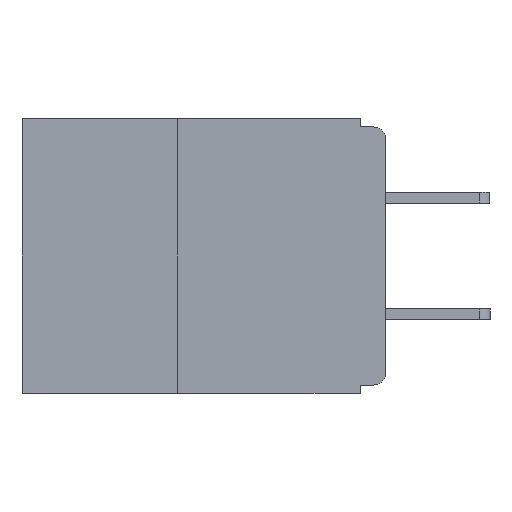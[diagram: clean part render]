
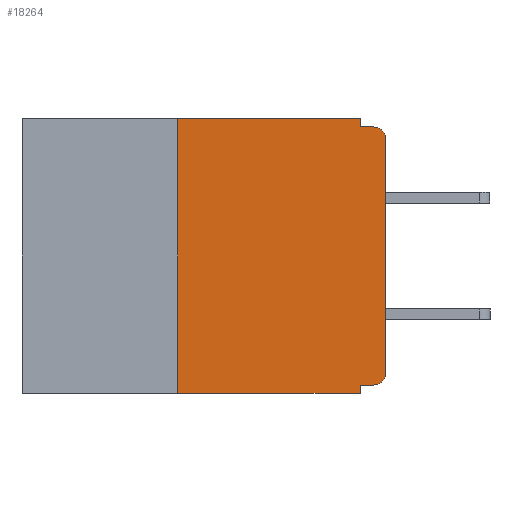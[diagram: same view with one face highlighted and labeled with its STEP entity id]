
A CAD part, left-side view. The second image highlights one B-rep face of the part: STEP entity #18264.
In plain terms, the highlighted planar face has unit normal (-1, 0, 0).
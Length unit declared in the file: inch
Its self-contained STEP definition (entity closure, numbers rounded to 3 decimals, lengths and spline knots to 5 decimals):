
#257 = VECTOR ( 'NONE', #6056, 39.37008 ) ;
#702 = CARTESIAN_POINT ( 'NONE',  ( 0., 0., -0.32 ) ) ;
#811 = EDGE_CURVE ( 'NONE', #17630, #2903, #16535, .T. ) ;
#1136 = ORIENTED_EDGE ( 'NONE', *, *, #19101, .F. ) ;
#1212 = DIRECTION ( 'NONE',  ( 0., 0., -1. ) ) ;
#1790 = CIRCLE ( 'NONE', #14953, 0.015 ) ;
#2903 = VERTEX_POINT ( 'NONE', #19510 ) ;
#2907 = VECTOR ( 'NONE', #17362, 39.37008 ) ;
#3308 = ORIENTED_EDGE ( 'NONE', *, *, #12771, .F. ) ;
#3456 = ORIENTED_EDGE ( 'NONE', *, *, #5571, .T. ) ;
#3699 = CARTESIAN_POINT ( 'NONE',  ( 0., 0.015, -0.01 ) ) ;
#4176 = VERTEX_POINT ( 'NONE', #11591 ) ;
#4193 = CARTESIAN_POINT ( 'NONE',  ( 0., 0., -0.025 ) ) ;
#4346 = CARTESIAN_POINT ( 'NONE',  ( 0., 0.031, -0.33 ) ) ;
#4763 = CARTESIAN_POINT ( 'NONE',  ( 0., 0.031, 0. ) ) ;
#5239 = AXIS2_PLACEMENT_3D ( 'NONE', #20608, #12041, #1212 ) ;
#5341 = CARTESIAN_POINT ( 'NONE',  ( 0., 0.015, -0.32 ) ) ;
#5507 = LINE ( 'NONE', #16270, #18462 ) ;
#5552 = DIRECTION ( 'NONE',  ( 0., -1., 0. ) ) ;
#5571 = EDGE_CURVE ( 'NONE', #7308, #18471, #18989, .T. ) ;
#6011 = CARTESIAN_POINT ( 'NONE',  ( 0., 0., 0. ) ) ;
#6017 = EDGE_CURVE ( 'NONE', #15058, #17630, #14954, .T. ) ;
#6056 = DIRECTION ( 'NONE',  ( 0., 0., 1. ) ) ;
#6274 = CARTESIAN_POINT ( 'NONE',  ( 0., 0.015, -0.025 ) ) ;
#6986 = CARTESIAN_POINT ( 'NONE',  ( 0., 0.25, -0.33 ) ) ;
#7021 = CARTESIAN_POINT ( 'NONE',  ( 0., 0.25, -0.33 ) ) ;
#7308 = VERTEX_POINT ( 'NONE', #5341 ) ;
#7648 = ORIENTED_EDGE ( 'NONE', *, *, #6017, .F. ) ;
#7984 = DIRECTION ( 'NONE',  ( 0., 1., 0. ) ) ;
#8058 = LINE ( 'NONE', #6986, #21852 ) ;
#8125 = DIRECTION ( 'NONE',  ( 0., 0., -1. ) ) ;
#8219 = VECTOR ( 'NONE', #7984, 39.37008 ) ;
#8510 = ORIENTED_EDGE ( 'NONE', *, *, #8783, .T. ) ;
#8783 = EDGE_CURVE ( 'NONE', #18471, #19861, #19153, .T. ) ;
#8837 = DIRECTION ( 'NONE',  ( 0., 0., 1. ) ) ;
#9544 = VERTEX_POINT ( 'NONE', #7021 ) ;
#10381 = EDGE_CURVE ( 'NONE', #19861, #16102, #1790, .T. ) ;
#10534 = VECTOR ( 'NONE', #5552, 39.37008 ) ;
#10900 = CARTESIAN_POINT ( 'NONE',  ( 0., 0., -0.01 ) ) ;
#11591 = CARTESIAN_POINT ( 'NONE',  ( 0., 0.031, -0.32 ) ) ;
#11940 = DIRECTION ( 'NONE',  ( 0., 0., -1. ) ) ;
#11958 = DIRECTION ( 'NONE',  ( -1., 0., 0. ) ) ;
#12041 = DIRECTION ( 'NONE',  ( 1., 0., 0. ) ) ;
#12095 = CARTESIAN_POINT ( 'NONE',  ( 0., 0.015, -0.305 ) ) ;
#12771 = EDGE_CURVE ( 'NONE', #7308, #4176, #17525, .T. ) ;
#13008 = LINE ( 'NONE', #19274, #21551 ) ;
#13403 = VERTEX_POINT ( 'NONE', #4346 ) ;
#13596 = CARTESIAN_POINT ( 'NONE',  ( 0., 0.031, 0. ) ) ;
#13736 = ORIENTED_EDGE ( 'NONE', *, *, #811, .F. ) ;
#14538 = DIRECTION ( 'NONE',  ( 0., 0., -1. ) ) ;
#14953 = AXIS2_PLACEMENT_3D ( 'NONE', #6274, #18572, #8125 ) ;
#14954 = LINE ( 'NONE', #22426, #18971 ) ;
#15058 = VERTEX_POINT ( 'NONE', #21295 ) ;
#15749 = LINE ( 'NONE', #10900, #10534 ) ;
#16102 = VERTEX_POINT ( 'NONE', #3699 ) ;
#16140 = CARTESIAN_POINT ( 'NONE',  ( 0., 0., -0.305 ) ) ;
#16270 = CARTESIAN_POINT ( 'NONE',  ( 0., 0.031, -0.33 ) ) ;
#16535 = LINE ( 'NONE', #4763, #2907 ) ;
#17181 = AXIS2_PLACEMENT_3D ( 'NONE', #12095, #11958, #11940 ) ;
#17362 = DIRECTION ( 'NONE',  ( 0., 0., -1. ) ) ;
#17525 = LINE ( 'NONE', #702, #8219 ) ;
#17569 = DIRECTION ( 'NONE',  ( 0., -1., 0. ) ) ;
#17630 = VERTEX_POINT ( 'NONE', #13596 ) ;
#17760 = EDGE_LOOP ( 'NONE', ( #8510, #17808, #18863, #13736, #7648, #21473, #22542, #1136, #3308, #3456 ) ) ;
#17808 = ORIENTED_EDGE ( 'NONE', *, *, #10381, .T. ) ;
#18264 = ADVANCED_FACE ( 'NONE', ( #22451 ), #22298, .F. ) ;
#18462 = VECTOR ( 'NONE', #14538, 39.37008 ) ;
#18471 = VERTEX_POINT ( 'NONE', #16140 ) ;
#18572 = DIRECTION ( 'NONE',  ( -1., 0., 0. ) ) ;
#18863 = ORIENTED_EDGE ( 'NONE', *, *, #19675, .F. ) ;
#18971 = VECTOR ( 'NONE', #22571, 39.37008 ) ;
#18989 = CIRCLE ( 'NONE', #17181, 0.015 ) ;
#19101 = EDGE_CURVE ( 'NONE', #4176, #13403, #5507, .T. ) ;
#19153 = LINE ( 'NONE', #6011, #257 ) ;
#19274 = CARTESIAN_POINT ( 'NONE',  ( 0., 0.437, -0.33 ) ) ;
#19510 = CARTESIAN_POINT ( 'NONE',  ( 0., 0.031, -0.01 ) ) ;
#19675 = EDGE_CURVE ( 'NONE', #2903, #16102, #15749, .T. ) ;
#19861 = VERTEX_POINT ( 'NONE', #4193 ) ;
#20233 = EDGE_CURVE ( 'NONE', #9544, #13403, #13008, .T. ) ;
#20608 = CARTESIAN_POINT ( 'NONE',  ( 0., 0.437, 0. ) ) ;
#21295 = CARTESIAN_POINT ( 'NONE',  ( 0., 0.25, 0. ) ) ;
#21473 = ORIENTED_EDGE ( 'NONE', *, *, #22486, .F. ) ;
#21551 = VECTOR ( 'NONE', #17569, 39.37008 ) ;
#21852 = VECTOR ( 'NONE', #8837, 39.37008 ) ;
#22298 = PLANE ( 'NONE',  #5239 ) ;
#22426 = CARTESIAN_POINT ( 'NONE',  ( 0., 0.437, 0. ) ) ;
#22451 = FACE_OUTER_BOUND ( 'NONE', #17760, .T. ) ;
#22486 = EDGE_CURVE ( 'NONE', #9544, #15058, #8058, .T. ) ;
#22542 = ORIENTED_EDGE ( 'NONE', *, *, #20233, .T. ) ;
#22571 = DIRECTION ( 'NONE',  ( 0., -1., 0. ) ) ;
